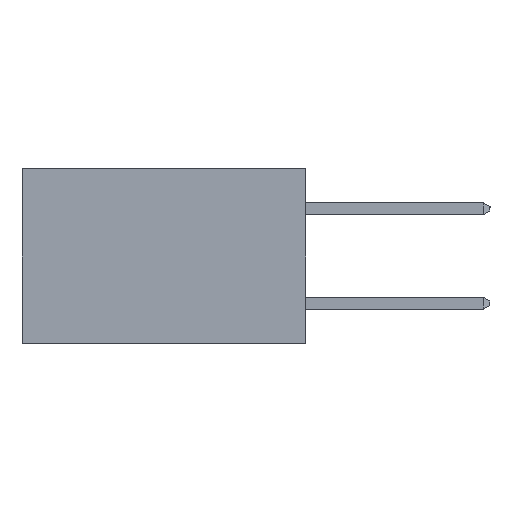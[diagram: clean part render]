
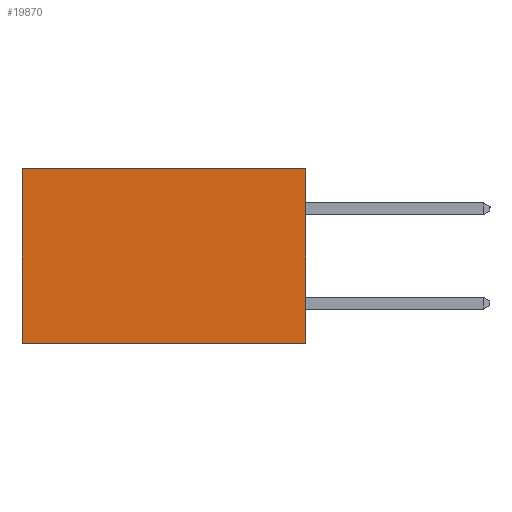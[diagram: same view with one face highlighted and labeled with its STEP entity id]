
A CAD part, left-side view. The second image highlights one B-rep face of the part: STEP entity #19870.
In plain terms, the highlighted planar face has unit normal (-1, 0, 0).
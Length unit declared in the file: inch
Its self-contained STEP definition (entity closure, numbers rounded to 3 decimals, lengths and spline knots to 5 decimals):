
#1530 = DIRECTION ( 'NONE',  ( 0., 1., 0. ) ) ;
#2990 = VERTEX_POINT ( 'NONE', #19348 ) ;
#3480 = VECTOR ( 'NONE', #24233, 39.37008 ) ;
#3566 = CARTESIAN_POINT ( 'NONE',  ( 0.2615, 0.6, -0.37 ) ) ;
#4300 = VERTEX_POINT ( 'NONE', #22937 ) ;
#4482 = CARTESIAN_POINT ( 'NONE',  ( 0.2615, 0., 0. ) ) ;
#5250 = VERTEX_POINT ( 'NONE', #3566 ) ;
#9752 = DIRECTION ( 'NONE',  ( 0., 1., 0. ) ) ;
#10120 = LINE ( 'NONE', #23125, #15415 ) ;
#10182 = DIRECTION ( 'NONE',  ( 0., 0., -1. ) ) ;
#11111 = ORIENTED_EDGE ( 'NONE', *, *, #12463, .F. ) ;
#11243 = LINE ( 'NONE', #20369, #3480 ) ;
#12373 = VECTOR ( 'NONE', #1530, 39.37008 ) ;
#12463 = EDGE_CURVE ( 'NONE', #4300, #5250, #10120, .T. ) ;
#13381 = EDGE_CURVE ( 'NONE', #2990, #5250, #16411, .T. ) ;
#13997 = AXIS2_PLACEMENT_3D ( 'NONE', #17928, #16064, #10182 ) ;
#15415 = VECTOR ( 'NONE', #9752, 39.37008 ) ;
#15597 = VERTEX_POINT ( 'NONE', #4482 ) ;
#15688 = EDGE_CURVE ( 'NONE', #15597, #4300, #11243, .T. ) ;
#15756 = ORIENTED_EDGE ( 'NONE', *, *, #15688, .F. ) ;
#16064 = DIRECTION ( 'NONE',  ( 1., 0., 0. ) ) ;
#16176 = PLANE ( 'NONE',  #13997 ) ;
#16411 = LINE ( 'NONE', #18146, #20603 ) ;
#17811 = ORIENTED_EDGE ( 'NONE', *, *, #13381, .T. ) ;
#17928 = CARTESIAN_POINT ( 'NONE',  ( 0.2615, 0., -0.37 ) ) ;
#18146 = CARTESIAN_POINT ( 'NONE',  ( 0.2615, 0.6, -0.37 ) ) ;
#18938 = LINE ( 'NONE', #24320, #12373 ) ;
#19348 = CARTESIAN_POINT ( 'NONE',  ( 0.2615, 0.6, 0. ) ) ;
#19509 = EDGE_CURVE ( 'NONE', #15597, #2990, #18938, .T. ) ;
#19775 = DIRECTION ( 'NONE',  ( 0., 0., -1. ) ) ;
#19870 = ADVANCED_FACE ( 'NONE', ( #21554 ), #16176, .F. ) ;
#20369 = CARTESIAN_POINT ( 'NONE',  ( 0.2615, 0., -0.37 ) ) ;
#20603 = VECTOR ( 'NONE', #19775, 39.37008 ) ;
#21554 = FACE_OUTER_BOUND ( 'NONE', #22924, .T. ) ;
#22924 = EDGE_LOOP ( 'NONE', ( #17811, #11111, #15756, #23041 ) ) ;
#22937 = CARTESIAN_POINT ( 'NONE',  ( 0.2615, 0., -0.37 ) ) ;
#23041 = ORIENTED_EDGE ( 'NONE', *, *, #19509, .T. ) ;
#23125 = CARTESIAN_POINT ( 'NONE',  ( 0.2615, 0., -0.37 ) ) ;
#24233 = DIRECTION ( 'NONE',  ( 0., 0., -1. ) ) ;
#24320 = CARTESIAN_POINT ( 'NONE',  ( 0.2615, 0., 0. ) ) ;
